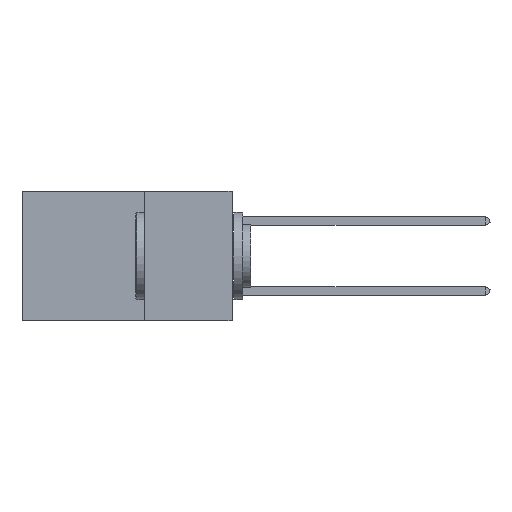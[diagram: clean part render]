
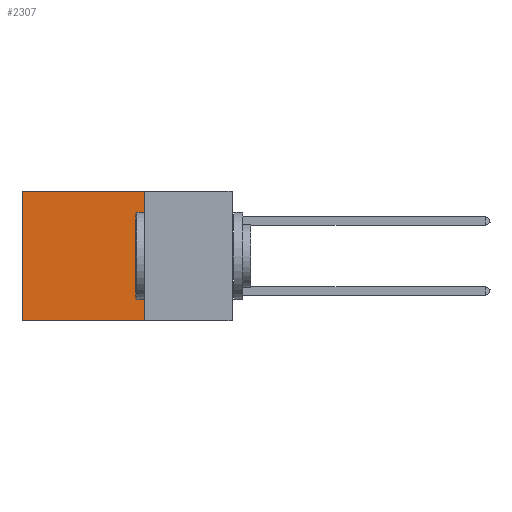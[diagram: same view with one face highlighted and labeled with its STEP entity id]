
A CAD part, left-side view. The second image highlights one B-rep face of the part: STEP entity #2307.
In plain terms, the highlighted planar face has unit normal (-1, 0, 0).
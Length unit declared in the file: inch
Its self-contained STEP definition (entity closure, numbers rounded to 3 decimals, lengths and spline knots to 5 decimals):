
#398 = CARTESIAN_POINT ( 'NONE',  ( 0.2875, 0.25, -0.37 ) ) ;
#2307 = ADVANCED_FACE ( 'NONE', ( #15511 ), #14103, .F. ) ;
#2456 = EDGE_CURVE ( 'NONE', #29149, #2591, #11028, .T. ) ;
#2591 = VERTEX_POINT ( 'NONE', #8559 ) ;
#4702 = VECTOR ( 'NONE', #28852, 39.37008 ) ;
#5249 = CARTESIAN_POINT ( 'NONE',  ( 0.2875, 0.6, 0. ) ) ;
#5474 = VECTOR ( 'NONE', #7541, 39.37008 ) ;
#6570 = LINE ( 'NONE', #12337, #5474 ) ;
#7231 = CARTESIAN_POINT ( 'NONE',  ( 0.2875, 0.25, -0.37 ) ) ;
#7541 = DIRECTION ( 'NONE',  ( 0., 1., 0. ) ) ;
#8559 = CARTESIAN_POINT ( 'NONE',  ( 0.2875, 0.6, -0.37 ) ) ;
#10541 = DIRECTION ( 'NONE',  ( 1., 0., 0. ) ) ;
#11028 = LINE ( 'NONE', #398, #4702 ) ;
#11312 = ORIENTED_EDGE ( 'NONE', *, *, #2456, .F. ) ;
#11913 = ORIENTED_EDGE ( 'NONE', *, *, #12414, .F. ) ;
#12337 = CARTESIAN_POINT ( 'NONE',  ( 0.2875, 0.25, 0. ) ) ;
#12414 = EDGE_CURVE ( 'NONE', #20825, #29149, #20607, .T. ) ;
#13684 = VECTOR ( 'NONE', #19245, 39.37008 ) ;
#13884 = CARTESIAN_POINT ( 'NONE',  ( 0.2875, 0.25, 0. ) ) ;
#14103 = PLANE ( 'NONE',  #30125 ) ;
#15085 = CARTESIAN_POINT ( 'NONE',  ( 0.2875, 0.6, 0. ) ) ;
#15511 = FACE_OUTER_BOUND ( 'NONE', #27200, .T. ) ;
#16742 = ORIENTED_EDGE ( 'NONE', *, *, #30424, .T. ) ;
#18221 = CARTESIAN_POINT ( 'NONE',  ( 0.2875, 0.25, 0. ) ) ;
#19245 = DIRECTION ( 'NONE',  ( 0., 0., -1. ) ) ;
#20607 = LINE ( 'NONE', #18221, #30711 ) ;
#20825 = VERTEX_POINT ( 'NONE', #13884 ) ;
#22895 = DIRECTION ( 'NONE',  ( 0., 0., -1. ) ) ;
#24292 = DIRECTION ( 'NONE',  ( 0., 0., -1. ) ) ;
#25190 = EDGE_CURVE ( 'NONE', #29878, #2591, #26025, .T. ) ;
#26025 = LINE ( 'NONE', #5249, #13684 ) ;
#26958 = CARTESIAN_POINT ( 'NONE',  ( 0.2875, 0.25, 0. ) ) ;
#27200 = EDGE_LOOP ( 'NONE', ( #27234, #11312, #11913, #16742 ) ) ;
#27234 = ORIENTED_EDGE ( 'NONE', *, *, #25190, .T. ) ;
#28852 = DIRECTION ( 'NONE',  ( 0., 1., 0. ) ) ;
#29149 = VERTEX_POINT ( 'NONE', #7231 ) ;
#29878 = VERTEX_POINT ( 'NONE', #15085 ) ;
#30125 = AXIS2_PLACEMENT_3D ( 'NONE', #26958, #10541, #24292 ) ;
#30424 = EDGE_CURVE ( 'NONE', #20825, #29878, #6570, .T. ) ;
#30711 = VECTOR ( 'NONE', #22895, 39.37008 ) ;
